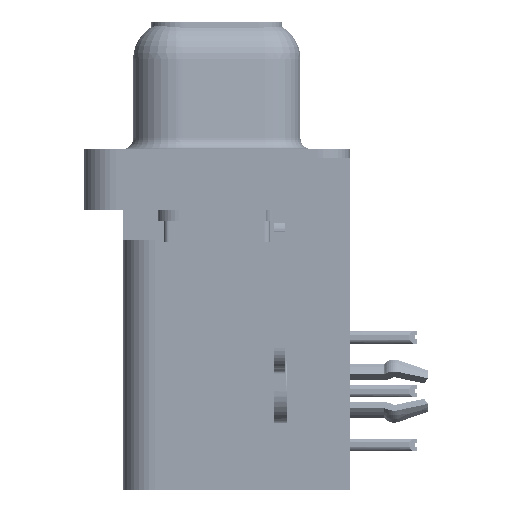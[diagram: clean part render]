
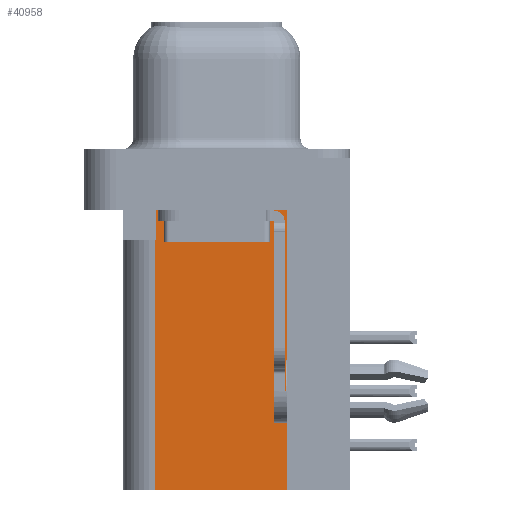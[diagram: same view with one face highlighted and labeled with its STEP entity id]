
A CAD part, left-side view. The second image highlights one B-rep face of the part: STEP entity #40958.
In plain terms, the highlighted planar face has unit normal (-1, 0, 0).
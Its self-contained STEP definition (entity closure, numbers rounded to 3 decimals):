
#1222 = PLANE ( 'NONE',  #25734 ) ;
#1337 = CARTESIAN_POINT ( 'NONE',  ( 3.7, 2.925, -15.7 ) ) ;
#4137 = VERTEX_POINT ( 'NONE', #30627 ) ;
#4911 = DIRECTION ( 'NONE',  ( 0., 0., -1. ) ) ;
#5759 = CARTESIAN_POINT ( 'NONE',  ( 3.7, -3.295, -15.7 ) ) ;
#6120 = VERTEX_POINT ( 'NONE', #1337 ) ;
#6581 = VECTOR ( 'NONE', #20255, 1000. ) ;
#10617 = ORIENTED_EDGE ( 'NONE', *, *, #20485, .T. ) ;
#11139 = DIRECTION ( 'NONE',  ( 0., 1., 0. ) ) ;
#11932 = CARTESIAN_POINT ( 'NONE',  ( 3.7, -3.295, -2.5 ) ) ;
#12384 = CARTESIAN_POINT ( 'NONE',  ( 3.7, 2.895, -3.9 ) ) ;
#12409 = CARTESIAN_POINT ( 'NONE',  ( 3.7, 2.895, -3.9 ) ) ;
#13727 = DIRECTION ( 'NONE',  ( 0., 1., 0. ) ) ;
#14253 = LINE ( 'NONE', #11932, #31314 ) ;
#14451 = LINE ( 'NONE', #12409, #33737 ) ;
#14799 = VERTEX_POINT ( 'NONE', #19521 ) ;
#16194 = CARTESIAN_POINT ( 'NONE',  ( 3.7, -3.295, -15.7 ) ) ;
#16467 = LINE ( 'NONE', #36491, #27314 ) ;
#16642 = VECTOR ( 'NONE', #34748, 1000. ) ;
#19233 = DIRECTION ( 'NONE',  ( 0., 1., 0. ) ) ;
#19361 = CARTESIAN_POINT ( 'NONE',  ( 3.7, -3.295, -15.7 ) ) ;
#19421 = CARTESIAN_POINT ( 'NONE',  ( 3.7, 2.895, -2.5 ) ) ;
#19521 = CARTESIAN_POINT ( 'NONE',  ( 3.7, -3.295, -2.5 ) ) ;
#20255 = DIRECTION ( 'NONE',  ( 0., 0., 1. ) ) ;
#20485 = EDGE_CURVE ( 'NONE', #44582, #4137, #16467, .T. ) ;
#21039 = VERTEX_POINT ( 'NONE', #19421 ) ;
#22043 = ORIENTED_EDGE ( 'NONE', *, *, #30761, .F. ) ;
#22825 = VERTEX_POINT ( 'NONE', #16194 ) ;
#25109 = ORIENTED_EDGE ( 'NONE', *, *, #41838, .T. ) ;
#25734 = AXIS2_PLACEMENT_3D ( 'NONE', #19361, #26676, #4911 ) ;
#26676 = DIRECTION ( 'NONE',  ( 1., 0., 0. ) ) ;
#27314 = VECTOR ( 'NONE', #11139, 1000. ) ;
#27843 = ORIENTED_EDGE ( 'NONE', *, *, #29852, .T. ) ;
#29055 = EDGE_LOOP ( 'NONE', ( #27843, #25109, #10617, #41008, #22043, #42912 ) ) ;
#29555 = VECTOR ( 'NONE', #13727, 1000. ) ;
#29852 = EDGE_CURVE ( 'NONE', #14799, #21039, #14253, .T. ) ;
#30627 = CARTESIAN_POINT ( 'NONE',  ( 3.7, 2.925, -3.9 ) ) ;
#30666 = LINE ( 'NONE', #31836, #29555 ) ;
#30761 = EDGE_CURVE ( 'NONE', #22825, #6120, #30666, .T. ) ;
#31314 = VECTOR ( 'NONE', #19233, 1000. ) ;
#31836 = CARTESIAN_POINT ( 'NONE',  ( 3.7, -3.295, -15.7 ) ) ;
#33737 = VECTOR ( 'NONE', #37780, 1000. ) ;
#33968 = FACE_OUTER_BOUND ( 'NONE', #29055, .T. ) ;
#34748 = DIRECTION ( 'NONE',  ( 0., 0., 1. ) ) ;
#34821 = EDGE_CURVE ( 'NONE', #6120, #4137, #43958, .T. ) ;
#36491 = CARTESIAN_POINT ( 'NONE',  ( 3.7, 0., -3.9 ) ) ;
#37780 = DIRECTION ( 'NONE',  ( 0., 0., -1. ) ) ;
#40958 = ADVANCED_FACE ( 'NONE', ( #33968 ), #1222, .F. ) ;
#41008 = ORIENTED_EDGE ( 'NONE', *, *, #34821, .F. ) ;
#41838 = EDGE_CURVE ( 'NONE', #21039, #44582, #14451, .T. ) ;
#42866 = EDGE_CURVE ( 'NONE', #22825, #14799, #45503, .T. ) ;
#42912 = ORIENTED_EDGE ( 'NONE', *, *, #42866, .T. ) ;
#43958 = LINE ( 'NONE', #45532, #6581 ) ;
#44582 = VERTEX_POINT ( 'NONE', #12384 ) ;
#45503 = LINE ( 'NONE', #5759, #16642 ) ;
#45532 = CARTESIAN_POINT ( 'NONE',  ( 3.7, 2.925, -15.7 ) ) ;
